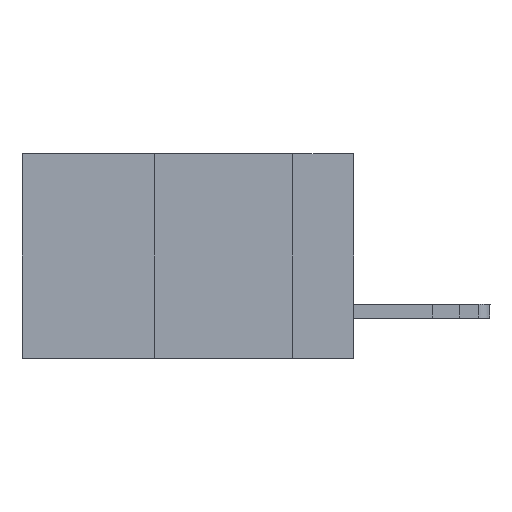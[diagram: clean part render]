
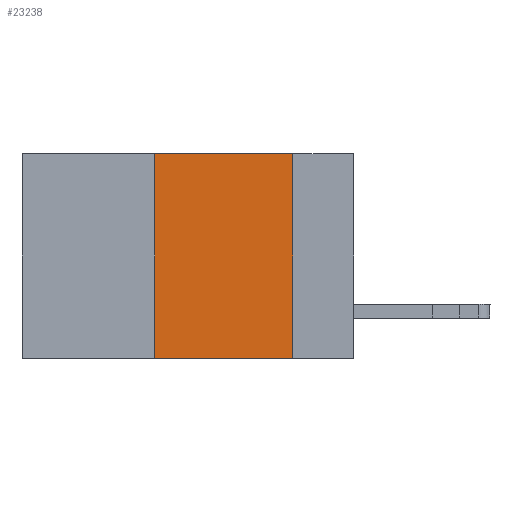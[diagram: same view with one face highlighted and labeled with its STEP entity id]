
A CAD part, left-side view. The second image highlights one B-rep face of the part: STEP entity #23238.
In plain terms, the highlighted planar face has unit normal (-1, 0, 0).
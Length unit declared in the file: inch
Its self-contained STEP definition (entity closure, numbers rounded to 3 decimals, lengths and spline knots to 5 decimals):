
#3444 = ORIENTED_EDGE ( 'NONE', *, *, #20901, .F. ) ;
#3588 = DIRECTION ( 'NONE',  ( 0., 0., -1. ) ) ;
#3814 = EDGE_CURVE ( 'NONE', #12756, #23807, #28011, .T. ) ;
#4305 = CARTESIAN_POINT ( 'NONE',  ( 0., 0.11, -0.37 ) ) ;
#4442 = LINE ( 'NONE', #4869, #27431 ) ;
#4628 = CARTESIAN_POINT ( 'NONE',  ( 0., 0.36, -0.37 ) ) ;
#4869 = CARTESIAN_POINT ( 'NONE',  ( 0., 0.6, -0.37 ) ) ;
#5215 = VECTOR ( 'NONE', #9865, 39.37008 ) ;
#5499 = ORIENTED_EDGE ( 'NONE', *, *, #24610, .F. ) ;
#5845 = VERTEX_POINT ( 'NONE', #4628 ) ;
#6681 = ORIENTED_EDGE ( 'NONE', *, *, #27346, .T. ) ;
#8429 = CARTESIAN_POINT ( 'NONE',  ( 0., 0.6, 0. ) ) ;
#9759 = VECTOR ( 'NONE', #23355, 39.37008 ) ;
#9865 = DIRECTION ( 'NONE',  ( 0., 0., 1. ) ) ;
#12756 = VERTEX_POINT ( 'NONE', #20084 ) ;
#13233 = DIRECTION ( 'NONE',  ( 0., -1., 0. ) ) ;
#13276 = ORIENTED_EDGE ( 'NONE', *, *, #3814, .F. ) ;
#13908 = FACE_OUTER_BOUND ( 'NONE', #13928, .T. ) ;
#13928 = EDGE_LOOP ( 'NONE', ( #3444, #13276, #5499, #6681 ) ) ;
#14543 = LINE ( 'NONE', #23372, #20670 ) ;
#14610 = LINE ( 'NONE', #23446, #5215 ) ;
#15647 = DIRECTION ( 'NONE',  ( 0., 0., -1. ) ) ;
#16079 = DIRECTION ( 'NONE',  ( 1., 0., 0. ) ) ;
#20084 = CARTESIAN_POINT ( 'NONE',  ( 0., 0.36, 0. ) ) ;
#20129 = CARTESIAN_POINT ( 'NONE',  ( 0., 0.6, 0. ) ) ;
#20670 = VECTOR ( 'NONE', #3588, 39.37008 ) ;
#20901 = EDGE_CURVE ( 'NONE', #23807, #27436, #14543, .T. ) ;
#23238 = ADVANCED_FACE ( 'NONE', ( #13908 ), #27378, .F. ) ;
#23355 = DIRECTION ( 'NONE',  ( 0., -1., 0. ) ) ;
#23372 = CARTESIAN_POINT ( 'NONE',  ( 0., 0.11, 0. ) ) ;
#23446 = CARTESIAN_POINT ( 'NONE',  ( 0., 0.36, 0. ) ) ;
#23807 = VERTEX_POINT ( 'NONE', #27923 ) ;
#24610 = EDGE_CURVE ( 'NONE', #5845, #12756, #14610, .T. ) ;
#26944 = AXIS2_PLACEMENT_3D ( 'NONE', #20129, #16079, #15647 ) ;
#27346 = EDGE_CURVE ( 'NONE', #5845, #27436, #4442, .T. ) ;
#27378 = PLANE ( 'NONE',  #26944 ) ;
#27431 = VECTOR ( 'NONE', #13233, 39.37008 ) ;
#27436 = VERTEX_POINT ( 'NONE', #4305 ) ;
#27923 = CARTESIAN_POINT ( 'NONE',  ( 0., 0.11, 0. ) ) ;
#28011 = LINE ( 'NONE', #8429, #9759 ) ;
